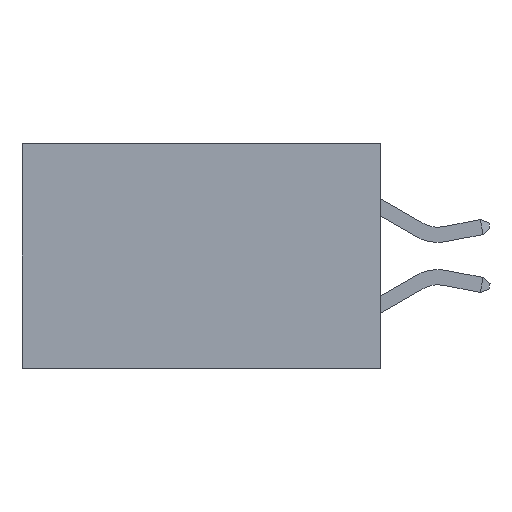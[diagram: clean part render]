
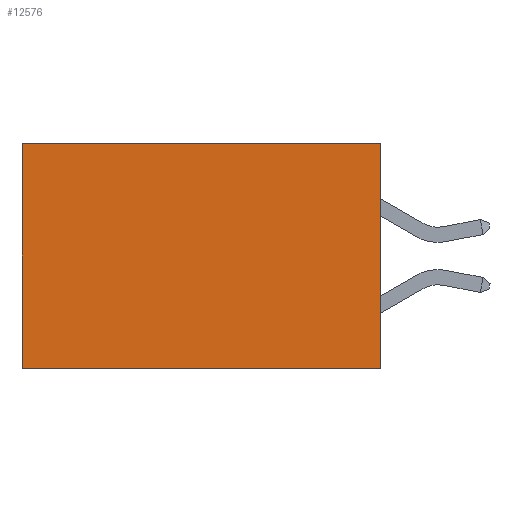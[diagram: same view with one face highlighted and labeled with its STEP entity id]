
A CAD part, left-side view. The second image highlights one B-rep face of the part: STEP entity #12576.
In plain terms, the highlighted planar face has unit normal (-1, 0, 0).
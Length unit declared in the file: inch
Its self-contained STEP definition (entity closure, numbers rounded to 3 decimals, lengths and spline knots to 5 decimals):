
#156 = DIRECTION ( 'NONE',  ( 0., 0., -1. ) ) ;
#1472 = ORIENTED_EDGE ( 'NONE', *, *, #4249, .T. ) ;
#1540 = CARTESIAN_POINT ( 'NONE',  ( 0.277, 0.59, 0. ) ) ;
#1816 = LINE ( 'NONE', #4553, #11056 ) ;
#2129 = CARTESIAN_POINT ( 'NONE',  ( 0.277, 0., -0.37 ) ) ;
#2569 = DIRECTION ( 'NONE',  ( 0., 1., 0. ) ) ;
#3238 = EDGE_CURVE ( 'NONE', #8459, #4756, #11116, .T. ) ;
#3555 = CARTESIAN_POINT ( 'NONE',  ( 0.277, 0., -0.37 ) ) ;
#3989 = EDGE_LOOP ( 'NONE', ( #1472, #8624, #12986, #4185 ) ) ;
#4185 = ORIENTED_EDGE ( 'NONE', *, *, #4325, .T. ) ;
#4188 = LINE ( 'NONE', #8132, #7274 ) ;
#4249 = EDGE_CURVE ( 'NONE', #12705, #4756, #1816, .T. ) ;
#4325 = EDGE_CURVE ( 'NONE', #5391, #12705, #4188, .T. ) ;
#4443 = DIRECTION ( 'NONE',  ( 0., 0., -1. ) ) ;
#4553 = CARTESIAN_POINT ( 'NONE',  ( 0.277, 0.59, -0.37 ) ) ;
#4756 = VERTEX_POINT ( 'NONE', #12902 ) ;
#4794 = PLANE ( 'NONE',  #9477 ) ;
#4991 = VECTOR ( 'NONE', #6503, 39.37008 ) ;
#5391 = VERTEX_POINT ( 'NONE', #10267 ) ;
#6503 = DIRECTION ( 'NONE',  ( 0., 1., 0. ) ) ;
#7076 = CARTESIAN_POINT ( 'NONE',  ( 0.277, 0., -0.37 ) ) ;
#7119 = DIRECTION ( 'NONE',  ( 1., 0., 0. ) ) ;
#7274 = VECTOR ( 'NONE', #2569, 39.37008 ) ;
#7997 = VECTOR ( 'NONE', #11651, 39.37008 ) ;
#8132 = CARTESIAN_POINT ( 'NONE',  ( 0.277, 0., 0. ) ) ;
#8459 = VERTEX_POINT ( 'NONE', #14917 ) ;
#8624 = ORIENTED_EDGE ( 'NONE', *, *, #3238, .F. ) ;
#9477 = AXIS2_PLACEMENT_3D ( 'NONE', #7076, #7119, #156 ) ;
#10267 = CARTESIAN_POINT ( 'NONE',  ( 0.277, 0., 0. ) ) ;
#11056 = VECTOR ( 'NONE', #4443, 39.37008 ) ;
#11073 = LINE ( 'NONE', #3555, #7997 ) ;
#11116 = LINE ( 'NONE', #2129, #4991 ) ;
#11651 = DIRECTION ( 'NONE',  ( 0., 0., -1. ) ) ;
#12576 = ADVANCED_FACE ( 'NONE', ( #14580 ), #4794, .F. ) ;
#12705 = VERTEX_POINT ( 'NONE', #1540 ) ;
#12902 = CARTESIAN_POINT ( 'NONE',  ( 0.277, 0.59, -0.37 ) ) ;
#12986 = ORIENTED_EDGE ( 'NONE', *, *, #13969, .F. ) ;
#13969 = EDGE_CURVE ( 'NONE', #5391, #8459, #11073, .T. ) ;
#14580 = FACE_OUTER_BOUND ( 'NONE', #3989, .T. ) ;
#14917 = CARTESIAN_POINT ( 'NONE',  ( 0.277, 0., -0.37 ) ) ;
